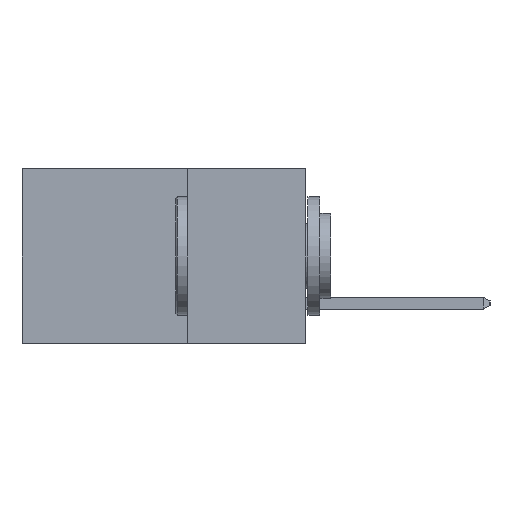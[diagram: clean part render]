
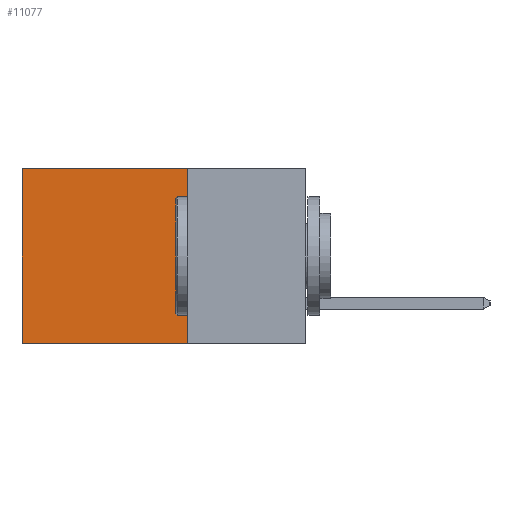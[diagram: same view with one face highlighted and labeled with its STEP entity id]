
A CAD part, left-side view. The second image highlights one B-rep face of the part: STEP entity #11077.
In plain terms, the highlighted planar face has unit normal (-1, 0, 0).
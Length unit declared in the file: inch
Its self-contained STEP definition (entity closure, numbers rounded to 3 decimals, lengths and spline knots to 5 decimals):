
#1728 = VECTOR ( 'NONE', #12079, 39.37008 ) ;
#1748 = VERTEX_POINT ( 'NONE', #10585 ) ;
#2368 = ORIENTED_EDGE ( 'NONE', *, *, #16744, .T. ) ;
#3247 = EDGE_CURVE ( 'NONE', #14912, #4258, #19754, .T. ) ;
#3326 = DIRECTION ( 'NONE',  ( 0., 1., 0. ) ) ;
#3345 = VECTOR ( 'NONE', #3326, 39.37008 ) ;
#3621 = EDGE_CURVE ( 'NONE', #1748, #4258, #8081, .T. ) ;
#3858 = CARTESIAN_POINT ( 'NONE',  ( 0.2615, 0.25, -0.37 ) ) ;
#4258 = VERTEX_POINT ( 'NONE', #7761 ) ;
#4832 = DIRECTION ( 'NONE',  ( 0., 0., -1. ) ) ;
#6161 = CARTESIAN_POINT ( 'NONE',  ( 0.2615, 0.25, -0.37 ) ) ;
#7068 = ORIENTED_EDGE ( 'NONE', *, *, #3247, .T. ) ;
#7243 = CARTESIAN_POINT ( 'NONE',  ( 0.2615, 0.25, -0.37 ) ) ;
#7761 = CARTESIAN_POINT ( 'NONE',  ( 0.2615, 0.6, -0.37 ) ) ;
#8081 = LINE ( 'NONE', #3858, #3345 ) ;
#8641 = CARTESIAN_POINT ( 'NONE',  ( 0.2615, 0.6, 0. ) ) ;
#10351 = LINE ( 'NONE', #6161, #19017 ) ;
#10585 = CARTESIAN_POINT ( 'NONE',  ( 0.2615, 0.25, -0.37 ) ) ;
#11077 = ADVANCED_FACE ( 'NONE', ( #18751 ), #11234, .F. ) ;
#11190 = DIRECTION ( 'NONE',  ( 0., 0., -1. ) ) ;
#11210 = DIRECTION ( 'NONE',  ( 1., 0., 0. ) ) ;
#11234 = PLANE ( 'NONE',  #16417 ) ;
#11252 = EDGE_CURVE ( 'NONE', #21015, #1748, #10351, .T. ) ;
#12079 = DIRECTION ( 'NONE',  ( 0., 0., -1. ) ) ;
#12107 = CARTESIAN_POINT ( 'NONE',  ( 0.2615, 0.6, -0.37 ) ) ;
#12182 = ORIENTED_EDGE ( 'NONE', *, *, #11252, .F. ) ;
#12638 = LINE ( 'NONE', #20451, #16710 ) ;
#13122 = ORIENTED_EDGE ( 'NONE', *, *, #3621, .F. ) ;
#13700 = DIRECTION ( 'NONE',  ( 0., 1., 0. ) ) ;
#14912 = VERTEX_POINT ( 'NONE', #8641 ) ;
#16417 = AXIS2_PLACEMENT_3D ( 'NONE', #7243, #11210, #11190 ) ;
#16710 = VECTOR ( 'NONE', #13700, 39.37008 ) ;
#16744 = EDGE_CURVE ( 'NONE', #21015, #14912, #12638, .T. ) ;
#18751 = FACE_OUTER_BOUND ( 'NONE', #22353, .T. ) ;
#19017 = VECTOR ( 'NONE', #4832, 39.37008 ) ;
#19754 = LINE ( 'NONE', #12107, #1728 ) ;
#19985 = CARTESIAN_POINT ( 'NONE',  ( 0.2615, 0.25, 0. ) ) ;
#20451 = CARTESIAN_POINT ( 'NONE',  ( 0.2615, 0.25, 0. ) ) ;
#21015 = VERTEX_POINT ( 'NONE', #19985 ) ;
#22353 = EDGE_LOOP ( 'NONE', ( #7068, #13122, #12182, #2368 ) ) ;
